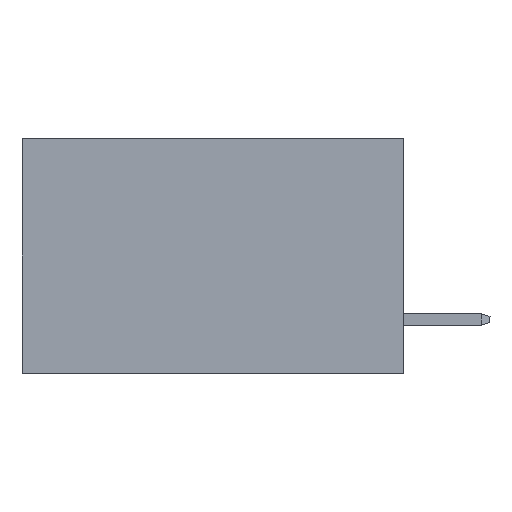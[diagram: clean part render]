
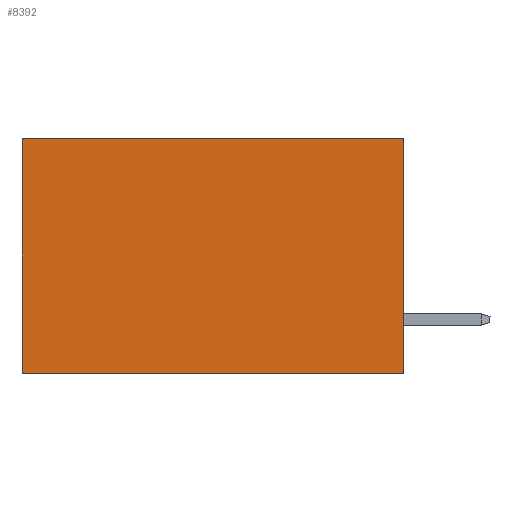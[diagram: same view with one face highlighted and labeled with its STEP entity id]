
A CAD part, left-side view. The second image highlights one B-rep face of the part: STEP entity #8392.
In plain terms, the highlighted planar face has unit normal (-1, 0, 0).
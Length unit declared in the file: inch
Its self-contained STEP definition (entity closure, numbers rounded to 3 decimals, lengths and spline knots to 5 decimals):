
#767 = DIRECTION ( 'NONE',  ( 0., 1., 0. ) ) ;
#1338 = CARTESIAN_POINT ( 'NONE',  ( 0.2875, 0.6, -0.37 ) ) ;
#1692 = VERTEX_POINT ( 'NONE', #5971 ) ;
#1778 = EDGE_LOOP ( 'NONE', ( #10687, #9691, #2104, #4844 ) ) ;
#1879 = LINE ( 'NONE', #6893, #6190 ) ;
#1968 = VECTOR ( 'NONE', #7472, 39.37008 ) ;
#2059 = VERTEX_POINT ( 'NONE', #1338 ) ;
#2104 = ORIENTED_EDGE ( 'NONE', *, *, #8294, .F. ) ;
#2210 = DIRECTION ( 'NONE',  ( 1., 0., 0. ) ) ;
#3342 = CARTESIAN_POINT ( 'NONE',  ( 0.2875, 0., -0.37 ) ) ;
#3459 = LINE ( 'NONE', #3342, #4472 ) ;
#3866 = FACE_OUTER_BOUND ( 'NONE', #1778, .T. ) ;
#3968 = CARTESIAN_POINT ( 'NONE',  ( 0.2875, 0.6, 0. ) ) ;
#4472 = VECTOR ( 'NONE', #767, 39.37008 ) ;
#4844 = ORIENTED_EDGE ( 'NONE', *, *, #5428, .T. ) ;
#4877 = VERTEX_POINT ( 'NONE', #8945 ) ;
#5428 = EDGE_CURVE ( 'NONE', #10816, #4877, #10705, .T. ) ;
#5729 = VECTOR ( 'NONE', #10641, 39.37008 ) ;
#5971 = CARTESIAN_POINT ( 'NONE',  ( 0.2875, 0., -0.37 ) ) ;
#6190 = VECTOR ( 'NONE', #10283, 39.37008 ) ;
#6440 = PLANE ( 'NONE',  #9580 ) ;
#6893 = CARTESIAN_POINT ( 'NONE',  ( 0.2875, 0., 0. ) ) ;
#7359 = CARTESIAN_POINT ( 'NONE',  ( 0.2875, 0., 0. ) ) ;
#7472 = DIRECTION ( 'NONE',  ( 0., 0., -1. ) ) ;
#7921 = LINE ( 'NONE', #3968, #1968 ) ;
#7941 = DIRECTION ( 'NONE',  ( 0., 0., -1. ) ) ;
#8294 = EDGE_CURVE ( 'NONE', #10816, #1692, #1879, .T. ) ;
#8392 = ADVANCED_FACE ( 'NONE', ( #3866 ), #6440, .F. ) ;
#8945 = CARTESIAN_POINT ( 'NONE',  ( 0.2875, 0.6, 0. ) ) ;
#8964 = CARTESIAN_POINT ( 'NONE',  ( 0.2875, 0., 0. ) ) ;
#9580 = AXIS2_PLACEMENT_3D ( 'NONE', #9836, #2210, #7941 ) ;
#9691 = ORIENTED_EDGE ( 'NONE', *, *, #10574, .F. ) ;
#9836 = CARTESIAN_POINT ( 'NONE',  ( 0.2875, 0., 0. ) ) ;
#10076 = EDGE_CURVE ( 'NONE', #4877, #2059, #7921, .T. ) ;
#10283 = DIRECTION ( 'NONE',  ( 0., 0., -1. ) ) ;
#10574 = EDGE_CURVE ( 'NONE', #1692, #2059, #3459, .T. ) ;
#10641 = DIRECTION ( 'NONE',  ( 0., 1., 0. ) ) ;
#10687 = ORIENTED_EDGE ( 'NONE', *, *, #10076, .T. ) ;
#10705 = LINE ( 'NONE', #7359, #5729 ) ;
#10816 = VERTEX_POINT ( 'NONE', #8964 ) ;
